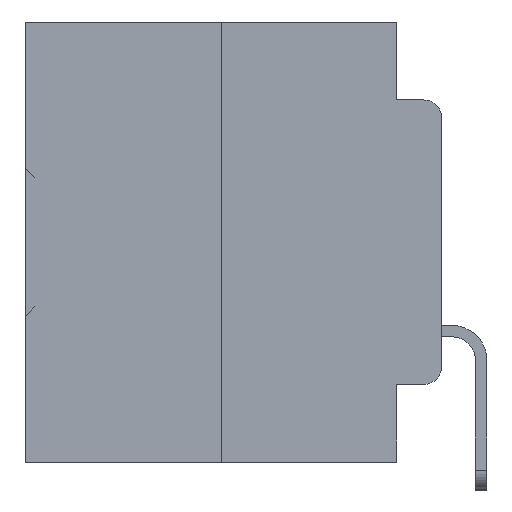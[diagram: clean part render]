
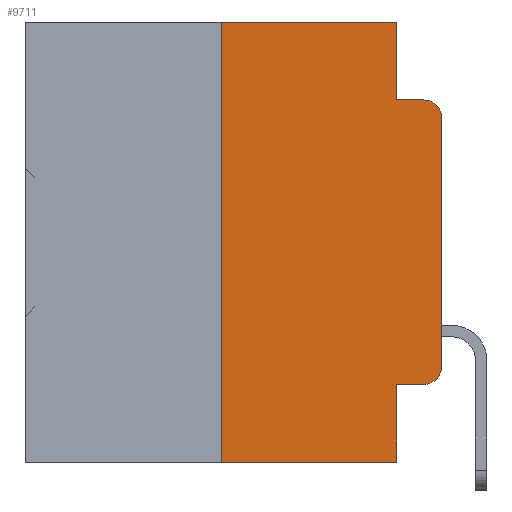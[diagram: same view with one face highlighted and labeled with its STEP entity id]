
A CAD part, left-side view. The second image highlights one B-rep face of the part: STEP entity #9711.
In plain terms, the highlighted planar face has unit normal (-1, 0, 0).
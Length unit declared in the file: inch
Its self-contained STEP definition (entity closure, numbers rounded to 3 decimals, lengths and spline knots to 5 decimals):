
#381 = VERTEX_POINT ( 'NONE', #8545 ) ;
#449 = LINE ( 'NONE', #35375, #6959 ) ;
#647 = VERTEX_POINT ( 'NONE', #16349 ) ;
#909 = EDGE_CURVE ( 'NONE', #30386, #21918, #2043, .T. ) ;
#1790 = CARTESIAN_POINT ( 'NONE',  ( 0., 0.051, 0. ) ) ;
#1843 = DIRECTION ( 'NONE',  ( 0., -1., 0. ) ) ;
#2043 = LINE ( 'NONE', #5761, #32096 ) ;
#3027 = LINE ( 'NONE', #13923, #33852 ) ;
#3650 = EDGE_CURVE ( 'NONE', #25796, #29945, #449, .T. ) ;
#3853 = AXIS2_PLACEMENT_3D ( 'NONE', #7420, #28284, #10554 ) ;
#4208 = ORIENTED_EDGE ( 'NONE', *, *, #27909, .T. ) ;
#4455 = VECTOR ( 'NONE', #1843, 39.37008 ) ;
#4575 = CARTESIAN_POINT ( 'NONE',  ( 0., 0.02, -0.0885 ) ) ;
#5030 = EDGE_CURVE ( 'NONE', #5545, #18136, #3027, .T. ) ;
#5545 = VERTEX_POINT ( 'NONE', #25341 ) ;
#5761 = CARTESIAN_POINT ( 'NONE',  ( 0., 0.051, 0. ) ) ;
#6959 = VECTOR ( 'NONE', #38195, 39.37008 ) ;
#7061 = LINE ( 'NONE', #23075, #13297 ) ;
#7119 = CARTESIAN_POINT ( 'NONE',  ( 0., 0., -0.3915 ) ) ;
#7343 = EDGE_CURVE ( 'NONE', #21918, #14286, #35966, .T. ) ;
#7420 = CARTESIAN_POINT ( 'NONE',  ( 0., 0.02, -0.3915 ) ) ;
#7627 = ORIENTED_EDGE ( 'NONE', *, *, #29224, .F. ) ;
#7859 = DIRECTION ( 'NONE',  ( 0., -1., 0. ) ) ;
#8545 = CARTESIAN_POINT ( 'NONE',  ( 0., 0.051, -0.4115 ) ) ;
#9563 = ORIENTED_EDGE ( 'NONE', *, *, #30028, .F. ) ;
#9683 = CARTESIAN_POINT ( 'NONE',  ( 0., 0.25, 0. ) ) ;
#9711 = ADVANCED_FACE ( 'NONE', ( #14787 ), #14219, .F. ) ;
#10180 = VECTOR ( 'NONE', #28446, 39.37008 ) ;
#10554 = DIRECTION ( 'NONE',  ( 0., 0., -1. ) ) ;
#10573 = CARTESIAN_POINT ( 'NONE',  ( 0., 0.051, 0. ) ) ;
#10635 = DIRECTION ( 'NONE',  ( 0., 0., -1. ) ) ;
#10736 = EDGE_CURVE ( 'NONE', #647, #25796, #37315, .T. ) ;
#11079 = DIRECTION ( 'NONE',  ( 0., -1., 0. ) ) ;
#11886 = AXIS2_PLACEMENT_3D ( 'NONE', #22524, #28367, #10635 ) ;
#12638 = CARTESIAN_POINT ( 'NONE',  ( 0., 0.051, -0.5 ) ) ;
#13297 = VECTOR ( 'NONE', #11079, 39.37008 ) ;
#13526 = EDGE_CURVE ( 'NONE', #29945, #14286, #36972, .T. ) ;
#13923 = CARTESIAN_POINT ( 'NONE',  ( 0., 0.473, -0.5 ) ) ;
#14219 = PLANE ( 'NONE',  #11886 ) ;
#14286 = VERTEX_POINT ( 'NONE', #4575 ) ;
#14502 = LINE ( 'NONE', #37745, #14734 ) ;
#14734 = VECTOR ( 'NONE', #20446, 39.37008 ) ;
#14787 = FACE_OUTER_BOUND ( 'NONE', #22879, .T. ) ;
#14807 = VERTEX_POINT ( 'NONE', #16325 ) ;
#15891 = DIRECTION ( 'NONE',  ( 0., 0., 1. ) ) ;
#16145 = CARTESIAN_POINT ( 'NONE',  ( 0., 0.02, -0.1085 ) ) ;
#16325 = CARTESIAN_POINT ( 'NONE',  ( 0., 0.25, 0. ) ) ;
#16349 = CARTESIAN_POINT ( 'NONE',  ( 0., 0.02, -0.4115 ) ) ;
#18136 = VERTEX_POINT ( 'NONE', #12638 ) ;
#18296 = LINE ( 'NONE', #10573, #10180 ) ;
#19093 = DIRECTION ( 'NONE',  ( 0., 0., -1. ) ) ;
#19991 = ORIENTED_EDGE ( 'NONE', *, *, #3650, .T. ) ;
#20446 = DIRECTION ( 'NONE',  ( 0., -1., 0. ) ) ;
#21918 = VERTEX_POINT ( 'NONE', #24256 ) ;
#22239 = EDGE_CURVE ( 'NONE', #381, #18136, #18296, .T. ) ;
#22524 = CARTESIAN_POINT ( 'NONE',  ( 0., 0.473, 0. ) ) ;
#22879 = EDGE_LOOP ( 'NONE', ( #19991, #35302, #28619, #30433, #7627, #9563, #25427, #27250, #4208, #29104 ) ) ;
#23075 = CARTESIAN_POINT ( 'NONE',  ( 0., 0.051, -0.4115 ) ) ;
#24256 = CARTESIAN_POINT ( 'NONE',  ( 0., 0.051, -0.0885 ) ) ;
#24301 = LINE ( 'NONE', #9683, #38583 ) ;
#25341 = CARTESIAN_POINT ( 'NONE',  ( 0., 0.25, -0.5 ) ) ;
#25427 = ORIENTED_EDGE ( 'NONE', *, *, #5030, .T. ) ;
#25796 = VERTEX_POINT ( 'NONE', #7119 ) ;
#26989 = CARTESIAN_POINT ( 'NONE',  ( 0., 0., -0.1085 ) ) ;
#27250 = ORIENTED_EDGE ( 'NONE', *, *, #22239, .F. ) ;
#27909 = EDGE_CURVE ( 'NONE', #381, #647, #7061, .T. ) ;
#28284 = DIRECTION ( 'NONE',  ( -1., 0., 0. ) ) ;
#28367 = DIRECTION ( 'NONE',  ( 1., 0., 0. ) ) ;
#28446 = DIRECTION ( 'NONE',  ( 0., 0., -1. ) ) ;
#28619 = ORIENTED_EDGE ( 'NONE', *, *, #7343, .F. ) ;
#28942 = CARTESIAN_POINT ( 'NONE',  ( 0., 0.051, -0.0885 ) ) ;
#29104 = ORIENTED_EDGE ( 'NONE', *, *, #10736, .T. ) ;
#29224 = EDGE_CURVE ( 'NONE', #14807, #30386, #14502, .T. ) ;
#29676 = DIRECTION ( 'NONE',  ( 0., 0., -1. ) ) ;
#29945 = VERTEX_POINT ( 'NONE', #26989 ) ;
#30028 = EDGE_CURVE ( 'NONE', #5545, #14807, #24301, .T. ) ;
#30386 = VERTEX_POINT ( 'NONE', #1790 ) ;
#30433 = ORIENTED_EDGE ( 'NONE', *, *, #909, .F. ) ;
#32096 = VECTOR ( 'NONE', #29676, 39.37008 ) ;
#33852 = VECTOR ( 'NONE', #7859, 39.37008 ) ;
#35302 = ORIENTED_EDGE ( 'NONE', *, *, #13526, .T. ) ;
#35375 = CARTESIAN_POINT ( 'NONE',  ( 0., 0., 0. ) ) ;
#35758 = AXIS2_PLACEMENT_3D ( 'NONE', #16145, #36325, #19093 ) ;
#35966 = LINE ( 'NONE', #28942, #4455 ) ;
#36325 = DIRECTION ( 'NONE',  ( -1., 0., 0. ) ) ;
#36972 = CIRCLE ( 'NONE', #35758, 0.02 ) ;
#37315 = CIRCLE ( 'NONE', #3853, 0.02 ) ;
#37745 = CARTESIAN_POINT ( 'NONE',  ( 0., 0.473, 0. ) ) ;
#38195 = DIRECTION ( 'NONE',  ( 0., 0., 1. ) ) ;
#38583 = VECTOR ( 'NONE', #15891, 39.37008 ) ;
